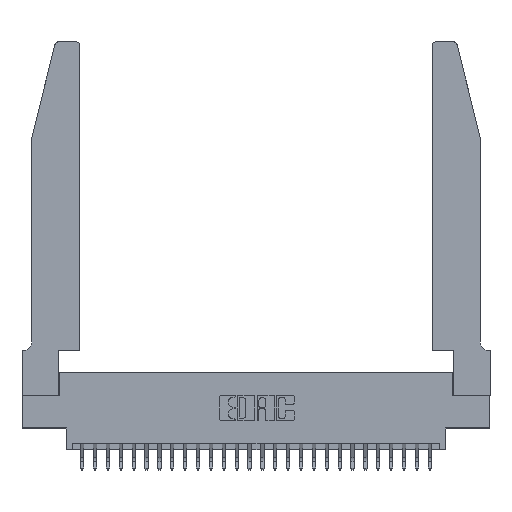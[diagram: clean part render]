
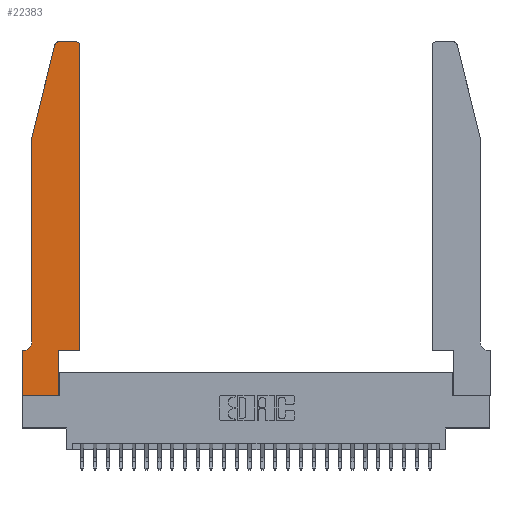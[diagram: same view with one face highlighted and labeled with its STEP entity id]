
A CAD part, top view. The second image highlights one B-rep face of the part: STEP entity #22383.
In plain terms, the highlighted planar face has unit normal (0, 0, 1).
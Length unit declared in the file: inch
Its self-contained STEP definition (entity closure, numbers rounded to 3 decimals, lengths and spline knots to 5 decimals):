
#204 = CARTESIAN_POINT ( 'NONE',  ( 0.0755, 2., 0.37 ) ) ;
#575 = PLANE ( 'NONE',  #2701 ) ;
#1521 = ORIENTED_EDGE ( 'NONE', *, *, #3939, .T. ) ;
#1800 = VECTOR ( 'NONE', #11561, 39.37008 ) ;
#2023 = VECTOR ( 'NONE', #28156, 39.37008 ) ;
#2305 = VERTEX_POINT ( 'NONE', #28842 ) ;
#2457 = EDGE_LOOP ( 'NONE', ( #27924, #1521, #5973, #21164, #20607, #12801, #11007, #22720, #20760, #19935, #22736, #19980 ) ) ;
#2701 = AXIS2_PLACEMENT_3D ( 'NONE', #2924, #18570, #16412 ) ;
#2727 = LINE ( 'NONE', #8416, #2023 ) ;
#2782 = VERTEX_POINT ( 'NONE', #11023 ) ;
#2924 = CARTESIAN_POINT ( 'NONE',  ( 0., 0.35, 0.37 ) ) ;
#3419 = VERTEX_POINT ( 'NONE', #24220 ) ;
#3745 = DIRECTION ( 'NONE',  ( -1., 0., 0. ) ) ;
#3939 = EDGE_CURVE ( 'NONE', #26389, #12839, #7479, .T. ) ;
#4148 = LINE ( 'NONE', #28734, #25450 ) ;
#4512 = DIRECTION ( 'NONE',  ( 1., 0., 0. ) ) ;
#4676 = DIRECTION ( 'NONE',  ( 0., 0., 1. ) ) ;
#5011 = VECTOR ( 'NONE', #17909, 39.37008 ) ;
#5561 = CIRCLE ( 'NONE', #23462, 0.03 ) ;
#5973 = ORIENTED_EDGE ( 'NONE', *, *, #20328, .T. ) ;
#6783 = CARTESIAN_POINT ( 'NONE',  ( 0.4505, 2.72, 0.37 ) ) ;
#7072 = DIRECTION ( 'NONE',  ( 1., 0., 0. ) ) ;
#7466 = LINE ( 'NONE', #27018, #24586 ) ;
#7479 = CIRCLE ( 'NONE', #28607, 0.03 ) ;
#7714 = EDGE_CURVE ( 'NONE', #10552, #26389, #7466, .T. ) ;
#8312 = EDGE_CURVE ( 'NONE', #13935, #24075, #19571, .T. ) ;
#8373 = VECTOR ( 'NONE', #21457, 39.37008 ) ;
#8416 = CARTESIAN_POINT ( 'NONE',  ( 0., 0., 0.37 ) ) ;
#8601 = CARTESIAN_POINT ( 'NONE',  ( 0., 0.35, 0.37 ) ) ;
#8652 = LINE ( 'NONE', #204, #18440 ) ;
#8997 = FACE_OUTER_BOUND ( 'NONE', #2457, .T. ) ;
#9000 = CARTESIAN_POINT ( 'NONE',  ( 0.0755, 2., 0.37 ) ) ;
#9140 = LINE ( 'NONE', #11467, #1800 ) ;
#10400 = LINE ( 'NONE', #26894, #24720 ) ;
#10552 = VERTEX_POINT ( 'NONE', #16960 ) ;
#10582 = CARTESIAN_POINT ( 'NONE',  ( 0.0055, 0.42, 0.37 ) ) ;
#10683 = CARTESIAN_POINT ( 'NONE',  ( 0., 0., 0.37 ) ) ;
#10723 = CARTESIAN_POINT ( 'NONE',  ( 0.0055, 0.35, 0.37 ) ) ;
#10938 = DIRECTION ( 'NONE',  ( 1., 0., 0. ) ) ;
#11007 = ORIENTED_EDGE ( 'NONE', *, *, #20152, .T. ) ;
#11023 = CARTESIAN_POINT ( 'NONE',  ( 0.4505, 0.35, 0.37 ) ) ;
#11422 = DIRECTION ( 'NONE',  ( 0., -1., 0. ) ) ;
#11467 = CARTESIAN_POINT ( 'NONE',  ( 0.4505, 0.35, 0.37 ) ) ;
#11561 = DIRECTION ( 'NONE',  ( 0., 1., 0. ) ) ;
#11990 = LINE ( 'NONE', #12996, #5011 ) ;
#11996 = DIRECTION ( 'NONE',  ( -0.239, -0.971, 0. ) ) ;
#12648 = AXIS2_PLACEMENT_3D ( 'NONE', #10582, #15086, #3745 ) ;
#12801 = ORIENTED_EDGE ( 'NONE', *, *, #8312, .T. ) ;
#12839 = VERTEX_POINT ( 'NONE', #16501 ) ;
#12878 = VECTOR ( 'NONE', #7072, 39.37008 ) ;
#12904 = CARTESIAN_POINT ( 'NONE',  ( 0.2865, 0.35, 0.37 ) ) ;
#12996 = CARTESIAN_POINT ( 'NONE',  ( 0.2865, 0.35, 0.37 ) ) ;
#13787 = EDGE_CURVE ( 'NONE', #2782, #28743, #9140, .T. ) ;
#13935 = VERTEX_POINT ( 'NONE', #10723 ) ;
#15086 = DIRECTION ( 'NONE',  ( 0., 0., -1. ) ) ;
#15352 = LINE ( 'NONE', #22726, #12878 ) ;
#15558 = VERTEX_POINT ( 'NONE', #9000 ) ;
#15656 = CARTESIAN_POINT ( 'NONE',  ( 0.284, 2.72, 0.37 ) ) ;
#16412 = DIRECTION ( 'NONE',  ( 1., 0., 0. ) ) ;
#16501 = CARTESIAN_POINT ( 'NONE',  ( 0.25487, 2.72718, 0.37 ) ) ;
#16960 = CARTESIAN_POINT ( 'NONE',  ( 0.4205, 2.75, 0.37 ) ) ;
#17909 = DIRECTION ( 'NONE',  ( 0., 1., 0. ) ) ;
#18153 = CARTESIAN_POINT ( 'NONE',  ( 0.4205, 2.72, 0.37 ) ) ;
#18440 = VECTOR ( 'NONE', #11996, 39.37008 ) ;
#18570 = DIRECTION ( 'NONE',  ( 0., 0., 1. ) ) ;
#18990 = CARTESIAN_POINT ( 'NONE',  ( 0.0755, 0.35, 0.37 ) ) ;
#19571 = LINE ( 'NONE', #18990, #8373 ) ;
#19599 = EDGE_CURVE ( 'NONE', #23466, #3419, #4148, .T. ) ;
#19935 = ORIENTED_EDGE ( 'NONE', *, *, #21670, .T. ) ;
#19959 = DIRECTION ( 'NONE',  ( 0., 0., 1. ) ) ;
#19980 = ORIENTED_EDGE ( 'NONE', *, *, #21048, .T. ) ;
#20152 = EDGE_CURVE ( 'NONE', #24075, #23466, #2727, .T. ) ;
#20328 = EDGE_CURVE ( 'NONE', #12839, #15558, #8652, .T. ) ;
#20607 = ORIENTED_EDGE ( 'NONE', *, *, #25220, .T. ) ;
#20760 = ORIENTED_EDGE ( 'NONE', *, *, #25372, .T. ) ;
#20803 = CARTESIAN_POINT ( 'NONE',  ( 0.284, 2.75, 0.37 ) ) ;
#21048 = EDGE_CURVE ( 'NONE', #28743, #10552, #5561, .T. ) ;
#21151 = CIRCLE ( 'NONE', #12648, 0.07 ) ;
#21164 = ORIENTED_EDGE ( 'NONE', *, *, #22305, .T. ) ;
#21457 = DIRECTION ( 'NONE',  ( -1., 0., 0. ) ) ;
#21670 = EDGE_CURVE ( 'NONE', #23471, #2782, #15352, .T. ) ;
#22305 = EDGE_CURVE ( 'NONE', #15558, #2305, #10400, .T. ) ;
#22383 = ADVANCED_FACE ( 'NONE', ( #8997 ), #575, .T. ) ;
#22631 = DIRECTION ( 'NONE',  ( -1., 0., 0. ) ) ;
#22720 = ORIENTED_EDGE ( 'NONE', *, *, #19599, .T. ) ;
#22726 = CARTESIAN_POINT ( 'NONE',  ( 0.4505, 0.35, 0.37 ) ) ;
#22736 = ORIENTED_EDGE ( 'NONE', *, *, #13787, .T. ) ;
#22857 = DIRECTION ( 'NONE',  ( 1., 0., 0. ) ) ;
#23462 = AXIS2_PLACEMENT_3D ( 'NONE', #18153, #4676, #22857 ) ;
#23466 = VERTEX_POINT ( 'NONE', #10683 ) ;
#23471 = VERTEX_POINT ( 'NONE', #12904 ) ;
#24075 = VERTEX_POINT ( 'NONE', #8601 ) ;
#24220 = CARTESIAN_POINT ( 'NONE',  ( 0.2865, 0., 0.37 ) ) ;
#24586 = VECTOR ( 'NONE', #22631, 39.37008 ) ;
#24720 = VECTOR ( 'NONE', #11422, 39.37008 ) ;
#25220 = EDGE_CURVE ( 'NONE', #2305, #13935, #21151, .T. ) ;
#25372 = EDGE_CURVE ( 'NONE', #3419, #23471, #11990, .T. ) ;
#25450 = VECTOR ( 'NONE', #10938, 39.37008 ) ;
#26389 = VERTEX_POINT ( 'NONE', #20803 ) ;
#26894 = CARTESIAN_POINT ( 'NONE',  ( 0.0755, 2., 0.37 ) ) ;
#27018 = CARTESIAN_POINT ( 'NONE',  ( 0.2605, 2.75, 0.37 ) ) ;
#27924 = ORIENTED_EDGE ( 'NONE', *, *, #7714, .T. ) ;
#28156 = DIRECTION ( 'NONE',  ( 0., -1., 0. ) ) ;
#28607 = AXIS2_PLACEMENT_3D ( 'NONE', #15656, #19959, #4512 ) ;
#28734 = CARTESIAN_POINT ( 'NONE',  ( 0., 0., 0.37 ) ) ;
#28743 = VERTEX_POINT ( 'NONE', #6783 ) ;
#28842 = CARTESIAN_POINT ( 'NONE',  ( 0.0755, 0.42, 0.37 ) ) ;
